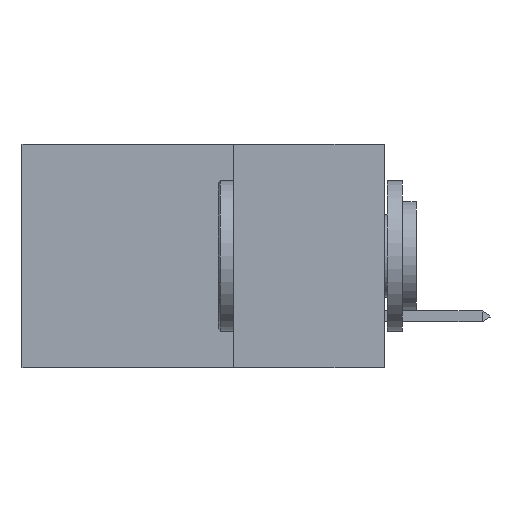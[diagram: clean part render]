
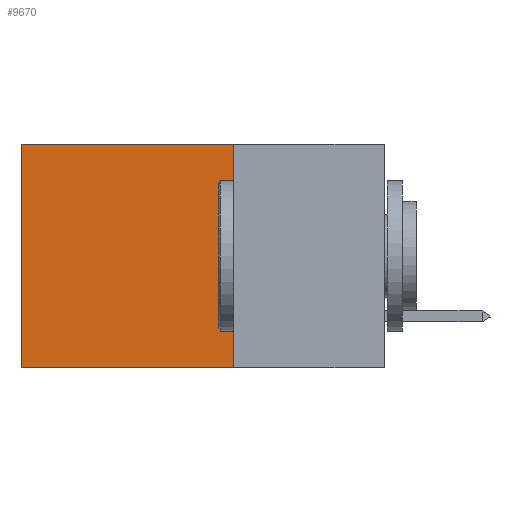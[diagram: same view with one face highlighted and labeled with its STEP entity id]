
A CAD part, left-side view. The second image highlights one B-rep face of the part: STEP entity #9670.
In plain terms, the highlighted planar face has unit normal (-1, 0, 0).
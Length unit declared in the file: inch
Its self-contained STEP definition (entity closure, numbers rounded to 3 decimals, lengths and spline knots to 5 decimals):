
#116 = CARTESIAN_POINT ( 'NONE',  ( 0.2875, 0.6, 0. ) ) ;
#252 = EDGE_CURVE ( 'NONE', #6736, #11336, #8657, .T. ) ;
#647 = DIRECTION ( 'NONE',  ( 0., 0., -1. ) ) ;
#845 = VECTOR ( 'NONE', #7533, 39.37008 ) ;
#1387 = EDGE_CURVE ( 'NONE', #4909, #11336, #6184, .T. ) ;
#1954 = ORIENTED_EDGE ( 'NONE', *, *, #252, .T. ) ;
#2619 = CARTESIAN_POINT ( 'NONE',  ( 0.2875, 0.25, 0. ) ) ;
#3092 = VECTOR ( 'NONE', #10160, 39.37008 ) ;
#3738 = VECTOR ( 'NONE', #11493, 39.37008 ) ;
#4516 = CARTESIAN_POINT ( 'NONE',  ( 0.2875, 0.6, -0.37 ) ) ;
#4909 = VERTEX_POINT ( 'NONE', #7673 ) ;
#4956 = CARTESIAN_POINT ( 'NONE',  ( 0.2875, 0.6, 0. ) ) ;
#5311 = DIRECTION ( 'NONE',  ( 1., 0., 0. ) ) ;
#5628 = VECTOR ( 'NONE', #5690, 39.37008 ) ;
#5690 = DIRECTION ( 'NONE',  ( 0., 0., -1. ) ) ;
#6184 = LINE ( 'NONE', #11173, #3738 ) ;
#6317 = PLANE ( 'NONE',  #10638 ) ;
#6736 = VERTEX_POINT ( 'NONE', #4956 ) ;
#7240 = EDGE_LOOP ( 'NONE', ( #1954, #11498, #10573, #11298 ) ) ;
#7360 = CARTESIAN_POINT ( 'NONE',  ( 0.2875, 0.25, 0. ) ) ;
#7526 = EDGE_CURVE ( 'NONE', #10744, #4909, #9759, .T. ) ;
#7533 = DIRECTION ( 'NONE',  ( 0., 1., 0. ) ) ;
#7673 = CARTESIAN_POINT ( 'NONE',  ( 0.2875, 0.25, -0.37 ) ) ;
#8657 = LINE ( 'NONE', #116, #5628 ) ;
#8811 = EDGE_CURVE ( 'NONE', #10744, #6736, #9516, .T. ) ;
#9516 = LINE ( 'NONE', #10323, #845 ) ;
#9670 = ADVANCED_FACE ( 'NONE', ( #11100 ), #6317, .F. ) ;
#9759 = LINE ( 'NONE', #7360, #3092 ) ;
#10160 = DIRECTION ( 'NONE',  ( 0., 0., -1. ) ) ;
#10323 = CARTESIAN_POINT ( 'NONE',  ( 0.2875, 0.25, 0. ) ) ;
#10573 = ORIENTED_EDGE ( 'NONE', *, *, #7526, .F. ) ;
#10638 = AXIS2_PLACEMENT_3D ( 'NONE', #2619, #5311, #647 ) ;
#10744 = VERTEX_POINT ( 'NONE', #11137 ) ;
#11100 = FACE_OUTER_BOUND ( 'NONE', #7240, .T. ) ;
#11137 = CARTESIAN_POINT ( 'NONE',  ( 0.2875, 0.25, 0. ) ) ;
#11173 = CARTESIAN_POINT ( 'NONE',  ( 0.2875, 0.25, -0.37 ) ) ;
#11298 = ORIENTED_EDGE ( 'NONE', *, *, #8811, .T. ) ;
#11336 = VERTEX_POINT ( 'NONE', #4516 ) ;
#11493 = DIRECTION ( 'NONE',  ( 0., 1., 0. ) ) ;
#11498 = ORIENTED_EDGE ( 'NONE', *, *, #1387, .F. ) ;
